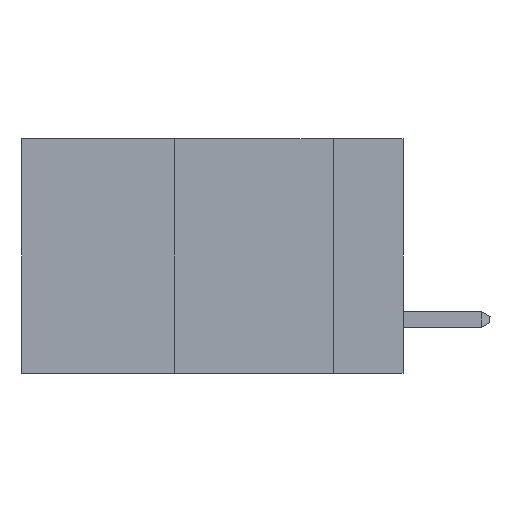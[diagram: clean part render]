
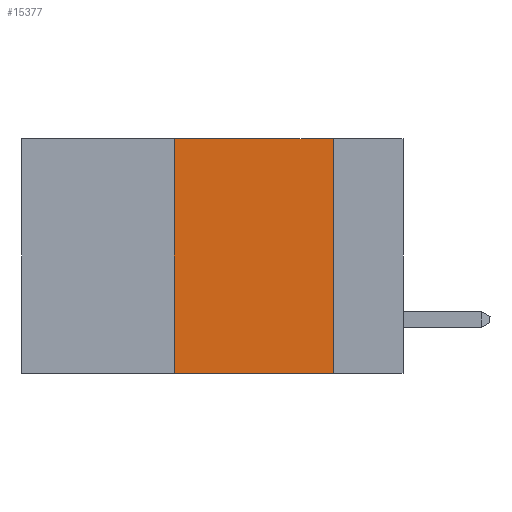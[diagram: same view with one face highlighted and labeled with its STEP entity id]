
A CAD part, left-side view. The second image highlights one B-rep face of the part: STEP entity #15377.
In plain terms, the highlighted planar face has unit normal (-1, 0, 0).
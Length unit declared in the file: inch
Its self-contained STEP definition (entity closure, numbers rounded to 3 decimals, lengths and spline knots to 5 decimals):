
#622 = DIRECTION ( 'NONE',  ( 0., 0., -1. ) ) ;
#1308 = DIRECTION ( 'NONE',  ( 0., 0., 1. ) ) ;
#1378 = LINE ( 'NONE', #7879, #9514 ) ;
#1441 = CARTESIAN_POINT ( 'NONE',  ( 0., 0.11, 0. ) ) ;
#2030 = ORIENTED_EDGE ( 'NONE', *, *, #3916, .F. ) ;
#2053 = VERTEX_POINT ( 'NONE', #13847 ) ;
#2133 = PLANE ( 'NONE',  #11048 ) ;
#2641 = VECTOR ( 'NONE', #3656, 39.37008 ) ;
#2711 = LINE ( 'NONE', #15503, #13457 ) ;
#2815 = CARTESIAN_POINT ( 'NONE',  ( 0., 0.36, 0. ) ) ;
#3349 = EDGE_CURVE ( 'NONE', #13323, #11666, #9269, .T. ) ;
#3656 = DIRECTION ( 'NONE',  ( 0., -1., 0. ) ) ;
#3916 = EDGE_CURVE ( 'NONE', #5697, #2053, #1378, .T. ) ;
#3971 = DIRECTION ( 'NONE',  ( 0., -1., 0. ) ) ;
#3993 = VECTOR ( 'NONE', #1308, 39.37008 ) ;
#5697 = VERTEX_POINT ( 'NONE', #1441 ) ;
#5718 = CARTESIAN_POINT ( 'NONE',  ( 0., 0.36, -0.37 ) ) ;
#6546 = ORIENTED_EDGE ( 'NONE', *, *, #14531, .F. ) ;
#7646 = ORIENTED_EDGE ( 'NONE', *, *, #15132, .T. ) ;
#7879 = CARTESIAN_POINT ( 'NONE',  ( 0., 0.11, 0. ) ) ;
#8554 = FACE_OUTER_BOUND ( 'NONE', #11096, .T. ) ;
#9269 = LINE ( 'NONE', #2815, #3993 ) ;
#9514 = VECTOR ( 'NONE', #10424, 39.37008 ) ;
#9835 = CARTESIAN_POINT ( 'NONE',  ( 0., 0.6, 0. ) ) ;
#10192 = LINE ( 'NONE', #15274, #2641 ) ;
#10424 = DIRECTION ( 'NONE',  ( 0., 0., -1. ) ) ;
#11048 = AXIS2_PLACEMENT_3D ( 'NONE', #9835, #14937, #622 ) ;
#11096 = EDGE_LOOP ( 'NONE', ( #2030, #6546, #15750, #7646 ) ) ;
#11666 = VERTEX_POINT ( 'NONE', #15879 ) ;
#13323 = VERTEX_POINT ( 'NONE', #5718 ) ;
#13457 = VECTOR ( 'NONE', #3971, 39.37008 ) ;
#13847 = CARTESIAN_POINT ( 'NONE',  ( 0., 0.11, -0.37 ) ) ;
#14531 = EDGE_CURVE ( 'NONE', #11666, #5697, #2711, .T. ) ;
#14937 = DIRECTION ( 'NONE',  ( 1., 0., 0. ) ) ;
#15132 = EDGE_CURVE ( 'NONE', #13323, #2053, #10192, .T. ) ;
#15274 = CARTESIAN_POINT ( 'NONE',  ( 0., 0.6, -0.37 ) ) ;
#15377 = ADVANCED_FACE ( 'NONE', ( #8554 ), #2133, .F. ) ;
#15503 = CARTESIAN_POINT ( 'NONE',  ( 0., 0.6, 0. ) ) ;
#15750 = ORIENTED_EDGE ( 'NONE', *, *, #3349, .F. ) ;
#15879 = CARTESIAN_POINT ( 'NONE',  ( 0., 0.36, 0. ) ) ;
